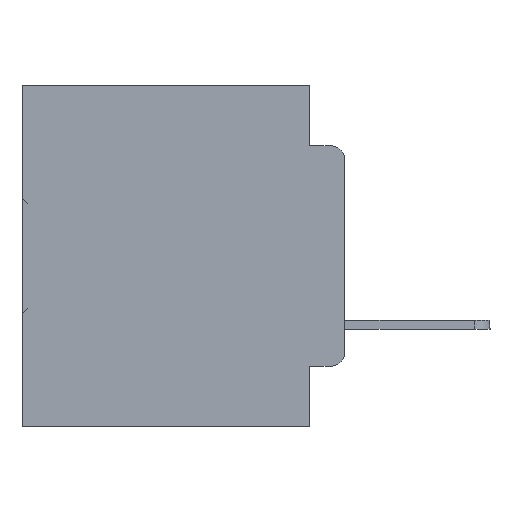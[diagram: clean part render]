
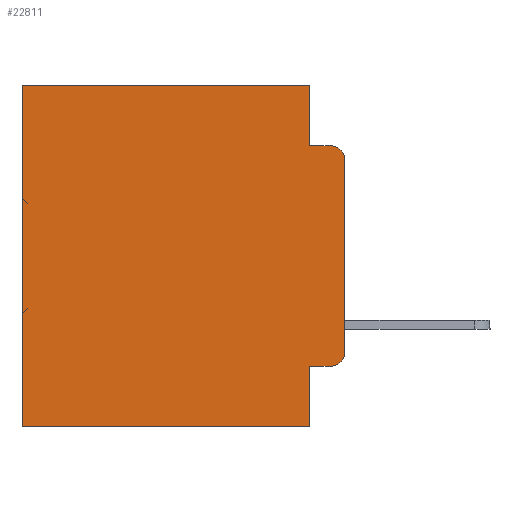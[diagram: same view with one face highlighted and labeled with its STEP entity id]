
A CAD part, left-side view. The second image highlights one B-rep face of the part: STEP entity #22811.
In plain terms, the highlighted planar face has unit normal (-1, 0, 0).
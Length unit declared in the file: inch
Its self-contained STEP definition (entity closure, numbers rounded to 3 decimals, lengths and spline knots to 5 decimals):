
#2225 = CIRCLE ( 'NONE', #25016, 0.02 ) ;
#2437 = CARTESIAN_POINT ( 'NONE',  ( 0.298, 0.473, 0. ) ) ;
#2488 = VERTEX_POINT ( 'NONE', #2676 ) ;
#2676 = CARTESIAN_POINT ( 'NONE',  ( 0.298, 0.051, -0.5 ) ) ;
#3299 = CARTESIAN_POINT ( 'NONE',  ( 0.298, 0.473, -0.5 ) ) ;
#3557 = CARTESIAN_POINT ( 'NONE',  ( 0.298, 0., -0.5 ) ) ;
#3575 = ORIENTED_EDGE ( 'NONE', *, *, #7277, .T. ) ;
#4617 = VERTEX_POINT ( 'NONE', #14261 ) ;
#5542 = CARTESIAN_POINT ( 'NONE',  ( 0.298, 0.02, -0.1085 ) ) ;
#6420 = LINE ( 'NONE', #9040, #36048 ) ;
#7277 = EDGE_CURVE ( 'NONE', #22098, #14484, #21103, .T. ) ;
#7755 = ORIENTED_EDGE ( 'NONE', *, *, #17264, .F. ) ;
#7958 = AXIS2_PLACEMENT_3D ( 'NONE', #5542, #22424, #24886 ) ;
#8153 = CARTESIAN_POINT ( 'NONE',  ( 0.298, 0.02, -0.3915 ) ) ;
#8486 = DIRECTION ( 'NONE',  ( 0., 0., -1. ) ) ;
#8795 = EDGE_CURVE ( 'NONE', #24367, #14484, #9843, .T. ) ;
#8850 = EDGE_CURVE ( 'NONE', #21125, #22281, #29575, .T. ) ;
#9020 = LINE ( 'NONE', #3557, #21419 ) ;
#9040 = CARTESIAN_POINT ( 'NONE',  ( 0.298, 0.051, 0. ) ) ;
#9249 = CARTESIAN_POINT ( 'NONE',  ( 0.298, 0., 0. ) ) ;
#9335 = EDGE_CURVE ( 'NONE', #22281, #30151, #36667, .T. ) ;
#9843 = LINE ( 'NONE', #15655, #32114 ) ;
#10739 = CARTESIAN_POINT ( 'NONE',  ( 0.298, 0., -0.3915 ) ) ;
#11353 = DIRECTION ( 'NONE',  ( -1., 0., 0. ) ) ;
#12428 = DIRECTION ( 'NONE',  ( 0., 0., -1. ) ) ;
#12724 = ORIENTED_EDGE ( 'NONE', *, *, #8850, .T. ) ;
#12867 = AXIS2_PLACEMENT_3D ( 'NONE', #9249, #15437, #12428 ) ;
#13172 = DIRECTION ( 'NONE',  ( 0., 0., -1. ) ) ;
#14261 = CARTESIAN_POINT ( 'NONE',  ( 0.298, 0.051, -0.4115 ) ) ;
#14323 = ORIENTED_EDGE ( 'NONE', *, *, #31010, .F. ) ;
#14484 = VERTEX_POINT ( 'NONE', #21944 ) ;
#15281 = DIRECTION ( 'NONE',  ( 0., 1., 0. ) ) ;
#15437 = DIRECTION ( 'NONE',  ( 1., 0., 0. ) ) ;
#15655 = CARTESIAN_POINT ( 'NONE',  ( 0.298, 0.051, -0.0885 ) ) ;
#17105 = CARTESIAN_POINT ( 'NONE',  ( 0.298, 0.02, -0.4115 ) ) ;
#17264 = EDGE_CURVE ( 'NONE', #4617, #2488, #6420, .T. ) ;
#17842 = DIRECTION ( 'NONE',  ( 0., 0., -1. ) ) ;
#18793 = ORIENTED_EDGE ( 'NONE', *, *, #19198, .F. ) ;
#18823 = DIRECTION ( 'NONE',  ( 0., -1., 0. ) ) ;
#19198 = EDGE_CURVE ( 'NONE', #21125, #24367, #22751, .T. ) ;
#19545 = LINE ( 'NONE', #25388, #35575 ) ;
#19587 = DIRECTION ( 'NONE',  ( 0., 0., -1. ) ) ;
#20127 = CARTESIAN_POINT ( 'NONE',  ( 0.298, 0.051, -0.0885 ) ) ;
#21103 = CIRCLE ( 'NONE', #7958, 0.02 ) ;
#21125 = VERTEX_POINT ( 'NONE', #26229 ) ;
#21166 = CARTESIAN_POINT ( 'NONE',  ( 0.298, 0., -0.1085 ) ) ;
#21419 = VECTOR ( 'NONE', #35489, 39.37008 ) ;
#21577 = VERTEX_POINT ( 'NONE', #10739 ) ;
#21756 = DIRECTION ( 'NONE',  ( 0., -1., 0. ) ) ;
#21944 = CARTESIAN_POINT ( 'NONE',  ( 0.298, 0.02, -0.0885 ) ) ;
#22098 = VERTEX_POINT ( 'NONE', #21166 ) ;
#22281 = VERTEX_POINT ( 'NONE', #22854 ) ;
#22312 = CARTESIAN_POINT ( 'NONE',  ( 0.298, 0.051, -0.4115 ) ) ;
#22424 = DIRECTION ( 'NONE',  ( -1., 0., 0. ) ) ;
#22470 = VECTOR ( 'NONE', #15281, 39.37008 ) ;
#22751 = LINE ( 'NONE', #34244, #33741 ) ;
#22811 = ADVANCED_FACE ( 'NONE', ( #32185 ), #27078, .F. ) ;
#22854 = CARTESIAN_POINT ( 'NONE',  ( 0.298, 0.473, 0. ) ) ;
#23435 = DIRECTION ( 'NONE',  ( 0., 0., -1. ) ) ;
#24367 = VERTEX_POINT ( 'NONE', #20127 ) ;
#24560 = EDGE_CURVE ( 'NONE', #4617, #37083, #36639, .T. ) ;
#24886 = DIRECTION ( 'NONE',  ( 0., 0., -1. ) ) ;
#25016 = AXIS2_PLACEMENT_3D ( 'NONE', #8153, #11353, #19587 ) ;
#25388 = CARTESIAN_POINT ( 'NONE',  ( 0.298, 0., 0. ) ) ;
#25651 = EDGE_CURVE ( 'NONE', #37083, #21577, #2225, .T. ) ;
#25980 = EDGE_CURVE ( 'NONE', #2488, #30151, #9020, .T. ) ;
#26229 = CARTESIAN_POINT ( 'NONE',  ( 0.298, 0.051, 0. ) ) ;
#26573 = ORIENTED_EDGE ( 'NONE', *, *, #8795, .F. ) ;
#27078 = PLANE ( 'NONE',  #12867 ) ;
#27341 = VECTOR ( 'NONE', #13172, 39.37008 ) ;
#28043 = EDGE_LOOP ( 'NONE', ( #14323, #3575, #26573, #18793, #12724, #34381, #35907, #7755, #28496, #33584 ) ) ;
#28496 = ORIENTED_EDGE ( 'NONE', *, *, #24560, .T. ) ;
#29575 = LINE ( 'NONE', #35393, #22470 ) ;
#30151 = VERTEX_POINT ( 'NONE', #3299 ) ;
#31010 = EDGE_CURVE ( 'NONE', #22098, #21577, #19545, .T. ) ;
#32114 = VECTOR ( 'NONE', #18823, 39.37008 ) ;
#32185 = FACE_OUTER_BOUND ( 'NONE', #28043, .T. ) ;
#33584 = ORIENTED_EDGE ( 'NONE', *, *, #25651, .T. ) ;
#33741 = VECTOR ( 'NONE', #8486, 39.37008 ) ;
#34244 = CARTESIAN_POINT ( 'NONE',  ( 0.298, 0.051, 0. ) ) ;
#34381 = ORIENTED_EDGE ( 'NONE', *, *, #9335, .T. ) ;
#35393 = CARTESIAN_POINT ( 'NONE',  ( 0.298, 0., 0. ) ) ;
#35489 = DIRECTION ( 'NONE',  ( 0., 1., 0. ) ) ;
#35575 = VECTOR ( 'NONE', #23435, 39.37008 ) ;
#35907 = ORIENTED_EDGE ( 'NONE', *, *, #25980, .F. ) ;
#36048 = VECTOR ( 'NONE', #17842, 39.37008 ) ;
#36390 = VECTOR ( 'NONE', #21756, 39.37008 ) ;
#36639 = LINE ( 'NONE', #22312, #36390 ) ;
#36667 = LINE ( 'NONE', #2437, #27341 ) ;
#37083 = VERTEX_POINT ( 'NONE', #17105 ) ;
